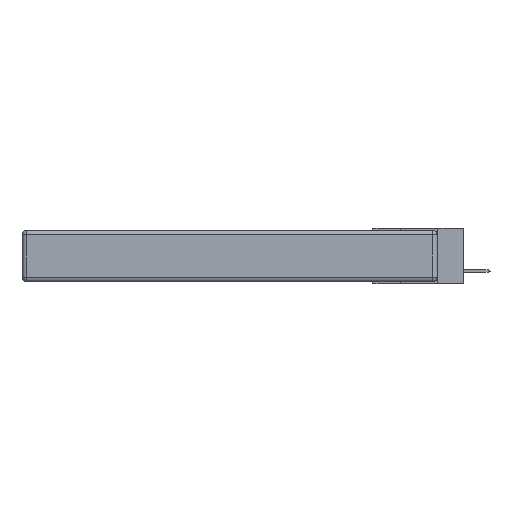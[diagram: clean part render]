
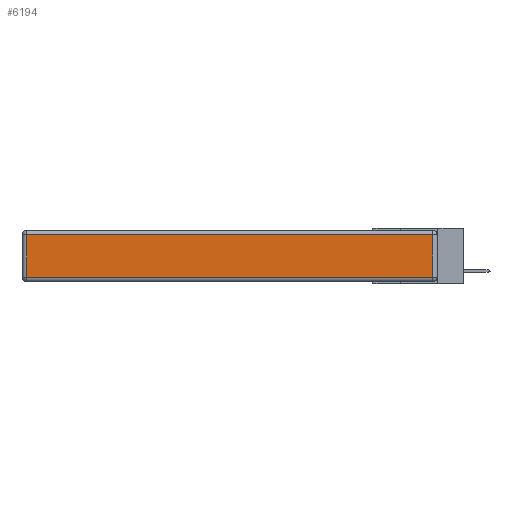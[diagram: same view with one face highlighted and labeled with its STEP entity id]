
A CAD part, left-side view. The second image highlights one B-rep face of the part: STEP entity #6194.
In plain terms, the highlighted planar face has unit normal (-1, 0, 0).
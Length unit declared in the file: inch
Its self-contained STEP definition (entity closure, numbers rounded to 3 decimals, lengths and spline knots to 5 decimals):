
#2771 = DIRECTION ( 'NONE',  ( 0., 1., 0. ) ) ;
#3769 = VERTEX_POINT ( 'NONE', #7481 ) ;
#3975 = CARTESIAN_POINT ( 'NONE',  ( 0., 2.72, -0.343 ) ) ;
#5008 = VECTOR ( 'NONE', #22462, 39.37008 ) ;
#5826 = DIRECTION ( 'NONE',  ( -1., 0., 0. ) ) ;
#6194 = ADVANCED_FACE ( 'NONE', ( #15330 ), #18745, .T. ) ;
#7481 = CARTESIAN_POINT ( 'NONE',  ( 0., 0.03, -0.03 ) ) ;
#7627 = VECTOR ( 'NONE', #8346, 39.37008 ) ;
#7793 = EDGE_LOOP ( 'NONE', ( #21098, #18815, #25282, #18193 ) ) ;
#7885 = CARTESIAN_POINT ( 'NONE',  ( 0., 2.72, -0.03 ) ) ;
#8308 = DIRECTION ( 'NONE',  ( 0., -1., 0. ) ) ;
#8346 = DIRECTION ( 'NONE',  ( 0., 0., -1. ) ) ;
#9270 = CARTESIAN_POINT ( 'NONE',  ( 0., 0.03, -0.313 ) ) ;
#9930 = VERTEX_POINT ( 'NONE', #7885 ) ;
#10107 = CARTESIAN_POINT ( 'NONE',  ( 0., 0., -0.343 ) ) ;
#10644 = VERTEX_POINT ( 'NONE', #9270 ) ;
#13002 = LINE ( 'NONE', #3975, #7627 ) ;
#13842 = CARTESIAN_POINT ( 'NONE',  ( 0., 2.72, -0.313 ) ) ;
#14375 = EDGE_CURVE ( 'NONE', #3769, #9930, #19339, .T. ) ;
#15330 = FACE_OUTER_BOUND ( 'NONE', #7793, .T. ) ;
#15406 = LINE ( 'NONE', #21292, #21479 ) ;
#17038 = EDGE_CURVE ( 'NONE', #10644, #3769, #26684, .T. ) ;
#18001 = VECTOR ( 'NONE', #2771, 39.37008 ) ;
#18137 = CARTESIAN_POINT ( 'NONE',  ( 0., 0.03, -0.343 ) ) ;
#18193 = ORIENTED_EDGE ( 'NONE', *, *, #19854, .T. ) ;
#18745 = PLANE ( 'NONE',  #20602 ) ;
#18815 = ORIENTED_EDGE ( 'NONE', *, *, #17038, .T. ) ;
#19339 = LINE ( 'NONE', #26529, #18001 ) ;
#19854 = EDGE_CURVE ( 'NONE', #9930, #25850, #13002, .T. ) ;
#20602 = AXIS2_PLACEMENT_3D ( 'NONE', #10107, #5826, #27495 ) ;
#21098 = ORIENTED_EDGE ( 'NONE', *, *, #21232, .T. ) ;
#21232 = EDGE_CURVE ( 'NONE', #25850, #10644, #15406, .T. ) ;
#21292 = CARTESIAN_POINT ( 'NONE',  ( 0., 0., -0.313 ) ) ;
#21479 = VECTOR ( 'NONE', #8308, 39.37008 ) ;
#22462 = DIRECTION ( 'NONE',  ( 0., 0., 1. ) ) ;
#25282 = ORIENTED_EDGE ( 'NONE', *, *, #14375, .T. ) ;
#25850 = VERTEX_POINT ( 'NONE', #13842 ) ;
#26529 = CARTESIAN_POINT ( 'NONE',  ( 0., 2.75, -0.03 ) ) ;
#26684 = LINE ( 'NONE', #18137, #5008 ) ;
#27495 = DIRECTION ( 'NONE',  ( 0., 0., 1. ) ) ;
